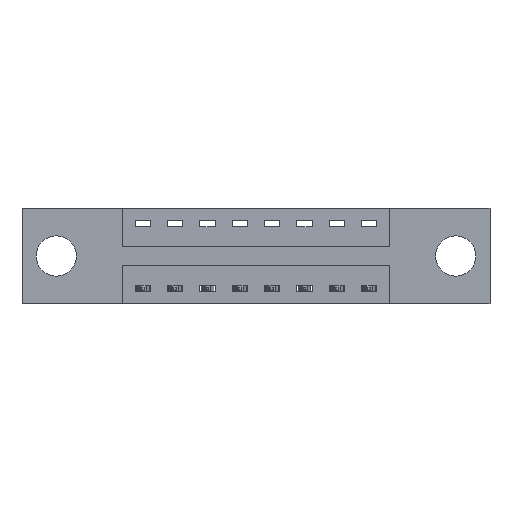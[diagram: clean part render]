
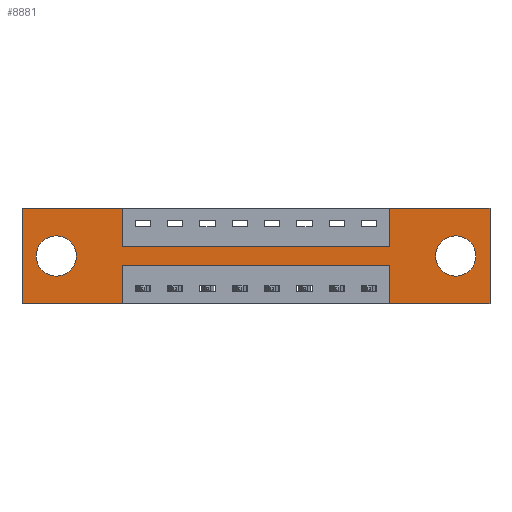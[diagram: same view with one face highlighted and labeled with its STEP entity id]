
A CAD part, front view. The second image highlights one B-rep face of the part: STEP entity #8881.
In plain terms, the highlighted planar face has unit normal (0, -1, 0).
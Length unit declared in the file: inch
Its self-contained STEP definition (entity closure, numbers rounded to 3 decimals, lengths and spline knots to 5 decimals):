
#3 = CARTESIAN_POINT ( 'NONE',  ( 1.6775, 0., -0.263 ) ) ;
#171 = CARTESIAN_POINT ( 'NONE',  ( 0.3875, 0., 0. ) ) ;
#196 = EDGE_CURVE ( 'NONE', #3524, #7320, #3985, .T. ) ;
#286 = EDGE_LOOP ( 'NONE', ( #506, #9245, #2881, #7753, #3863, #1694, #2477, #7693, #6750, #1043, #2927, #7834 ) ) ;
#423 = VECTOR ( 'NONE', #978, 39.37008 ) ;
#470 = DIRECTION ( 'NONE',  ( -1., 0., 0. ) ) ;
#493 = CARTESIAN_POINT ( 'NONE',  ( 1.81, 0., 0. ) ) ;
#494 = DIRECTION ( 'NONE',  ( 0., 0., 1. ) ) ;
#506 = ORIENTED_EDGE ( 'NONE', *, *, #6307, .F. ) ;
#535 = VERTEX_POINT ( 'NONE', #2922 ) ;
#553 = DIRECTION ( 'NONE',  ( 0., 0., 1. ) ) ;
#762 = CARTESIAN_POINT ( 'NONE',  ( 0., 0., 0. ) ) ;
#978 = DIRECTION ( 'NONE',  ( 0., 0., -1. ) ) ;
#1043 = ORIENTED_EDGE ( 'NONE', *, *, #9778, .F. ) ;
#1233 = DIRECTION ( 'NONE',  ( 0., 0., -1. ) ) ;
#1306 = LINE ( 'NONE', #8227, #3606 ) ;
#1411 = EDGE_CURVE ( 'NONE', #8057, #5478, #1489, .T. ) ;
#1418 = LINE ( 'NONE', #3003, #1660 ) ;
#1487 = CARTESIAN_POINT ( 'NONE',  ( 0.1325, 0., -0.185 ) ) ;
#1489 = LINE ( 'NONE', #9148, #9844 ) ;
#1528 = DIRECTION ( 'NONE',  ( 0., 1., 0. ) ) ;
#1660 = VECTOR ( 'NONE', #5209, 39.37008 ) ;
#1694 = ORIENTED_EDGE ( 'NONE', *, *, #3743, .F. ) ;
#2129 = CARTESIAN_POINT ( 'NONE',  ( 1.81, 0., 0. ) ) ;
#2168 = VECTOR ( 'NONE', #8815, 39.37008 ) ;
#2215 = CARTESIAN_POINT ( 'NONE',  ( 0.1325, 0., -0.263 ) ) ;
#2365 = VERTEX_POINT ( 'NONE', #9770 ) ;
#2393 = VERTEX_POINT ( 'NONE', #8385 ) ;
#2447 = VERTEX_POINT ( 'NONE', #171 ) ;
#2477 = ORIENTED_EDGE ( 'NONE', *, *, #7709, .F. ) ;
#2496 = VECTOR ( 'NONE', #470, 39.37008 ) ;
#2504 = CARTESIAN_POINT ( 'NONE',  ( 1.6775, 0., -0.185 ) ) ;
#2553 = DIRECTION ( 'NONE',  ( 0., 0., -1. ) ) ;
#2726 = VECTOR ( 'NONE', #4875, 39.37008 ) ;
#2783 = VERTEX_POINT ( 'NONE', #5298 ) ;
#2875 = CARTESIAN_POINT ( 'NONE',  ( 0.3875, 0., -0.15 ) ) ;
#2881 = ORIENTED_EDGE ( 'NONE', *, *, #8034, .F. ) ;
#2922 = CARTESIAN_POINT ( 'NONE',  ( 0., 0., -0.37 ) ) ;
#2927 = ORIENTED_EDGE ( 'NONE', *, *, #3381, .F. ) ;
#2931 = LINE ( 'NONE', #9143, #5946 ) ;
#2939 = VERTEX_POINT ( 'NONE', #8666 ) ;
#2964 = DIRECTION ( 'NONE',  ( 0., 0., -1. ) ) ;
#3000 = ORIENTED_EDGE ( 'NONE', *, *, #3477, .T. ) ;
#3003 = CARTESIAN_POINT ( 'NONE',  ( 1.4225, 0., 0. ) ) ;
#3135 = CIRCLE ( 'NONE', #6548, 0.078 ) ;
#3270 = CARTESIAN_POINT ( 'NONE',  ( 1.4225, 0., -0.15 ) ) ;
#3292 = DIRECTION ( 'NONE',  ( 0., 0., 1. ) ) ;
#3349 = CARTESIAN_POINT ( 'NONE',  ( 0., 0., -0.37 ) ) ;
#3364 = LINE ( 'NONE', #493, #6048 ) ;
#3380 = DIRECTION ( 'NONE',  ( 0., 1., 0. ) ) ;
#3381 = EDGE_CURVE ( 'NONE', #535, #2939, #3778, .T. ) ;
#3477 = EDGE_CURVE ( 'NONE', #3771, #2783, #4463, .T. ) ;
#3524 = VERTEX_POINT ( 'NONE', #5695 ) ;
#3606 = VECTOR ( 'NONE', #553, 39.37008 ) ;
#3717 = DIRECTION ( 'NONE',  ( 1., 0., 0. ) ) ;
#3743 = EDGE_CURVE ( 'NONE', #4729, #5365, #7715, .T. ) ;
#3771 = VERTEX_POINT ( 'NONE', #3 ) ;
#3778 = LINE ( 'NONE', #762, #4384 ) ;
#3809 = VECTOR ( 'NONE', #3717, 39.37008 ) ;
#3863 = ORIENTED_EDGE ( 'NONE', *, *, #8497, .F. ) ;
#3985 = CIRCLE ( 'NONE', #9659, 0.078 ) ;
#4229 = CARTESIAN_POINT ( 'NONE',  ( 1.4225, 0., -0.22 ) ) ;
#4384 = VECTOR ( 'NONE', #8578, 39.37008 ) ;
#4398 = VECTOR ( 'NONE', #2964, 39.37008 ) ;
#4463 = CIRCLE ( 'NONE', #9644, 0.078 ) ;
#4655 = LINE ( 'NONE', #7944, #423 ) ;
#4693 = ORIENTED_EDGE ( 'NONE', *, *, #196, .T. ) ;
#4722 = VERTEX_POINT ( 'NONE', #6224 ) ;
#4729 = VERTEX_POINT ( 'NONE', #5458 ) ;
#4831 = LINE ( 'NONE', #5482, #2726 ) ;
#4862 = PLANE ( 'NONE',  #5102 ) ;
#4875 = DIRECTION ( 'NONE',  ( -1., 0., 0. ) ) ;
#4966 = DIRECTION ( 'NONE',  ( 0., -1., 0. ) ) ;
#5102 = AXIS2_PLACEMENT_3D ( 'NONE', #3349, #4966, #1233 ) ;
#5209 = DIRECTION ( 'NONE',  ( 0., 0., 1. ) ) ;
#5292 = AXIS2_PLACEMENT_3D ( 'NONE', #8261, #7450, #494 ) ;
#5298 = CARTESIAN_POINT ( 'NONE',  ( 1.6775, 0., -0.107 ) ) ;
#5365 = VERTEX_POINT ( 'NONE', #2129 ) ;
#5458 = CARTESIAN_POINT ( 'NONE',  ( 1.4225, 0., 0. ) ) ;
#5478 = VERTEX_POINT ( 'NONE', #5674 ) ;
#5482 = CARTESIAN_POINT ( 'NONE',  ( 0., 0., -0.37 ) ) ;
#5674 = CARTESIAN_POINT ( 'NONE',  ( 0.3875, 0., -0.22 ) ) ;
#5695 = CARTESIAN_POINT ( 'NONE',  ( 0.1325, 0., -0.107 ) ) ;
#5714 = FACE_BOUND ( 'NONE', #6607, .T. ) ;
#5911 = CARTESIAN_POINT ( 'NONE',  ( 0., 0., -0.37 ) ) ;
#5946 = VECTOR ( 'NONE', #5987, 39.37008 ) ;
#5987 = DIRECTION ( 'NONE',  ( 1., 0., 0. ) ) ;
#6048 = VECTOR ( 'NONE', #6462, 39.37008 ) ;
#6081 = ORIENTED_EDGE ( 'NONE', *, *, #9864, .T. ) ;
#6224 = CARTESIAN_POINT ( 'NONE',  ( 1.81, 0., -0.37 ) ) ;
#6307 = EDGE_CURVE ( 'NONE', #5478, #2393, #9878, .T. ) ;
#6462 = DIRECTION ( 'NONE',  ( 0., 0., -1. ) ) ;
#6548 = AXIS2_PLACEMENT_3D ( 'NONE', #9544, #9692, #9742 ) ;
#6607 = EDGE_LOOP ( 'NONE', ( #4693, #6081 ) ) ;
#6724 = CARTESIAN_POINT ( 'NONE',  ( 0., 0., 0. ) ) ;
#6750 = ORIENTED_EDGE ( 'NONE', *, *, #9127, .F. ) ;
#6922 = DIRECTION ( 'NONE',  ( -1., 0., 0. ) ) ;
#7242 = EDGE_LOOP ( 'NONE', ( #8858, #3000 ) ) ;
#7320 = VERTEX_POINT ( 'NONE', #2215 ) ;
#7450 = DIRECTION ( 'NONE',  ( 0., 1., 0. ) ) ;
#7559 = CARTESIAN_POINT ( 'NONE',  ( 0., 0., 0. ) ) ;
#7693 = ORIENTED_EDGE ( 'NONE', *, *, #9958, .F. ) ;
#7709 = EDGE_CURVE ( 'NONE', #7927, #4729, #1418, .T. ) ;
#7715 = LINE ( 'NONE', #7559, #3809 ) ;
#7753 = ORIENTED_EDGE ( 'NONE', *, *, #8270, .F. ) ;
#7834 = ORIENTED_EDGE ( 'NONE', *, *, #9526, .F. ) ;
#7927 = VERTEX_POINT ( 'NONE', #3270 ) ;
#7944 = CARTESIAN_POINT ( 'NONE',  ( 0.3875, 0., 0. ) ) ;
#8034 = EDGE_CURVE ( 'NONE', #2365, #8057, #1306, .T. ) ;
#8057 = VERTEX_POINT ( 'NONE', #4229 ) ;
#8201 = FACE_BOUND ( 'NONE', #7242, .T. ) ;
#8227 = CARTESIAN_POINT ( 'NONE',  ( 1.4225, 0., -0.37 ) ) ;
#8239 = LINE ( 'NONE', #5911, #2496 ) ;
#8261 = CARTESIAN_POINT ( 'NONE',  ( 0.1325, 0., -0.185 ) ) ;
#8270 = EDGE_CURVE ( 'NONE', #4722, #2365, #4831, .T. ) ;
#8385 = CARTESIAN_POINT ( 'NONE',  ( 0.3875, 0., -0.37 ) ) ;
#8465 = EDGE_CURVE ( 'NONE', #2783, #3771, #3135, .T. ) ;
#8497 = EDGE_CURVE ( 'NONE', #5365, #4722, #3364, .T. ) ;
#8538 = CIRCLE ( 'NONE', #5292, 0.078 ) ;
#8578 = DIRECTION ( 'NONE',  ( 0., 0., 1. ) ) ;
#8666 = CARTESIAN_POINT ( 'NONE',  ( 0., 0., 0. ) ) ;
#8746 = FACE_OUTER_BOUND ( 'NONE', #286, .T. ) ;
#8815 = DIRECTION ( 'NONE',  ( 1., 0., 0. ) ) ;
#8858 = ORIENTED_EDGE ( 'NONE', *, *, #8465, .T. ) ;
#8881 = ADVANCED_FACE ( 'NONE', ( #8201, #5714, #8746 ), #4862, .T. ) ;
#8958 = VERTEX_POINT ( 'NONE', #2875 ) ;
#9127 = EDGE_CURVE ( 'NONE', #2447, #8958, #4655, .T. ) ;
#9128 = CARTESIAN_POINT ( 'NONE',  ( 0.3875, 0., -0.37 ) ) ;
#9143 = CARTESIAN_POINT ( 'NONE',  ( 0.3875, 0., -0.15 ) ) ;
#9148 = CARTESIAN_POINT ( 'NONE',  ( 0.3875, 0., -0.22 ) ) ;
#9245 = ORIENTED_EDGE ( 'NONE', *, *, #1411, .F. ) ;
#9526 = EDGE_CURVE ( 'NONE', #2393, #535, #8239, .T. ) ;
#9544 = CARTESIAN_POINT ( 'NONE',  ( 1.6775, 0., -0.185 ) ) ;
#9644 = AXIS2_PLACEMENT_3D ( 'NONE', #2504, #3380, #2553 ) ;
#9659 = AXIS2_PLACEMENT_3D ( 'NONE', #1487, #1528, #3292 ) ;
#9692 = DIRECTION ( 'NONE',  ( 0., 1., 0. ) ) ;
#9742 = DIRECTION ( 'NONE',  ( 0., 0., -1. ) ) ;
#9745 = LINE ( 'NONE', #6724, #2168 ) ;
#9770 = CARTESIAN_POINT ( 'NONE',  ( 1.4225, 0., -0.37 ) ) ;
#9778 = EDGE_CURVE ( 'NONE', #2939, #2447, #9745, .T. ) ;
#9844 = VECTOR ( 'NONE', #6922, 39.37008 ) ;
#9864 = EDGE_CURVE ( 'NONE', #7320, #3524, #8538, .T. ) ;
#9878 = LINE ( 'NONE', #9128, #4398 ) ;
#9958 = EDGE_CURVE ( 'NONE', #8958, #7927, #2931, .T. ) ;
